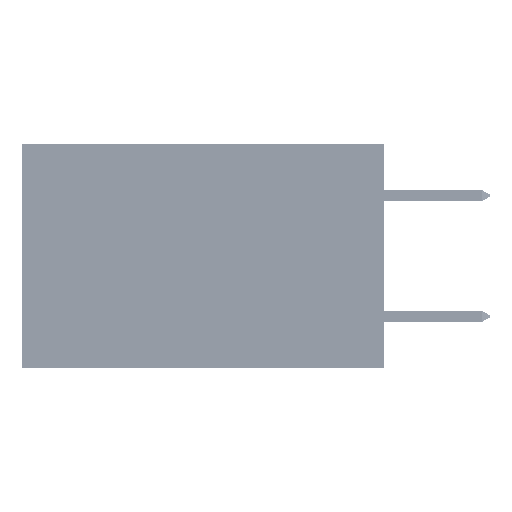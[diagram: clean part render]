
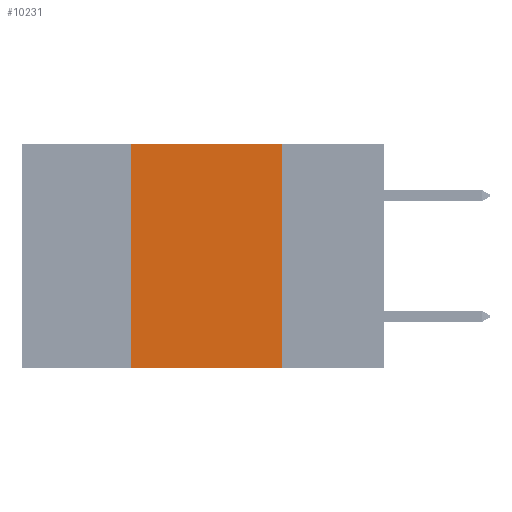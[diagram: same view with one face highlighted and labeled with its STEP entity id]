
A CAD part, left-side view. The second image highlights one B-rep face of the part: STEP entity #10231.
In plain terms, the highlighted planar face has unit normal (-1, 0, 0).
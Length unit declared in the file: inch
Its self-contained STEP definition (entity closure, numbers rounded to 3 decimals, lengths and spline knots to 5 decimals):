
#1757 = ORIENTED_EDGE ( 'NONE', *, *, #27164, .F. ) ;
#5419 = CARTESIAN_POINT ( 'NONE',  ( 0., 0.6, 0. ) ) ;
#5467 = VECTOR ( 'NONE', #23265, 39.37008 ) ;
#5619 = CARTESIAN_POINT ( 'NONE',  ( 0., 0.17, 0. ) ) ;
#6142 = EDGE_CURVE ( 'NONE', #15066, #35758, #28500, .T. ) ;
#8606 = DIRECTION ( 'NONE',  ( 0., 0., 1. ) ) ;
#9313 = PLANE ( 'NONE',  #13855 ) ;
#9495 = EDGE_LOOP ( 'NONE', ( #19611, #1757, #23736, #15697 ) ) ;
#10231 = ADVANCED_FACE ( 'NONE', ( #51678 ), #9313, .F. ) ;
#11993 = CARTESIAN_POINT ( 'NONE',  ( 0., 0.42, 0. ) ) ;
#12250 = VERTEX_POINT ( 'NONE', #31145 ) ;
#12843 = CARTESIAN_POINT ( 'NONE',  ( 0., 0.42, 0. ) ) ;
#13855 = AXIS2_PLACEMENT_3D ( 'NONE', #5419, #46111, #29637 ) ;
#14457 = CARTESIAN_POINT ( 'NONE',  ( 0., 0.42, -0.37 ) ) ;
#15066 = VERTEX_POINT ( 'NONE', #14457 ) ;
#15697 = ORIENTED_EDGE ( 'NONE', *, *, #6142, .T. ) ;
#17356 = DIRECTION ( 'NONE',  ( 0., 0., -1. ) ) ;
#17780 = VECTOR ( 'NONE', #8606, 39.37008 ) ;
#18787 = CARTESIAN_POINT ( 'NONE',  ( 0., 0.6, -0.37 ) ) ;
#19611 = ORIENTED_EDGE ( 'NONE', *, *, #42710, .F. ) ;
#19734 = CARTESIAN_POINT ( 'NONE',  ( 0., 0.6, 0. ) ) ;
#23265 = DIRECTION ( 'NONE',  ( 0., -1., 0. ) ) ;
#23362 = VECTOR ( 'NONE', #51010, 39.37008 ) ;
#23736 = ORIENTED_EDGE ( 'NONE', *, *, #47161, .F. ) ;
#25677 = LINE ( 'NONE', #5619, #42177 ) ;
#27164 = EDGE_CURVE ( 'NONE', #42422, #12250, #28368, .T. ) ;
#28368 = LINE ( 'NONE', #19734, #5467 ) ;
#28500 = LINE ( 'NONE', #18787, #23362 ) ;
#29637 = DIRECTION ( 'NONE',  ( 0., 0., -1. ) ) ;
#29919 = LINE ( 'NONE', #12843, #17780 ) ;
#31145 = CARTESIAN_POINT ( 'NONE',  ( 0., 0.17, 0. ) ) ;
#35758 = VERTEX_POINT ( 'NONE', #52486 ) ;
#42177 = VECTOR ( 'NONE', #17356, 39.37008 ) ;
#42422 = VERTEX_POINT ( 'NONE', #11993 ) ;
#42710 = EDGE_CURVE ( 'NONE', #12250, #35758, #25677, .T. ) ;
#46111 = DIRECTION ( 'NONE',  ( 1., 0., 0. ) ) ;
#47161 = EDGE_CURVE ( 'NONE', #15066, #42422, #29919, .T. ) ;
#51010 = DIRECTION ( 'NONE',  ( 0., -1., 0. ) ) ;
#51678 = FACE_OUTER_BOUND ( 'NONE', #9495, .T. ) ;
#52486 = CARTESIAN_POINT ( 'NONE',  ( 0., 0.17, -0.37 ) ) ;
